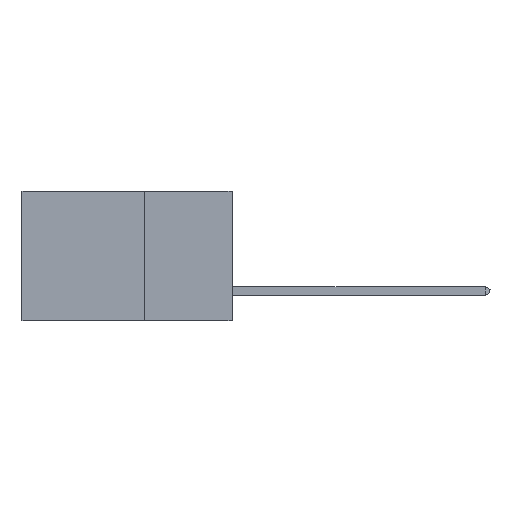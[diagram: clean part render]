
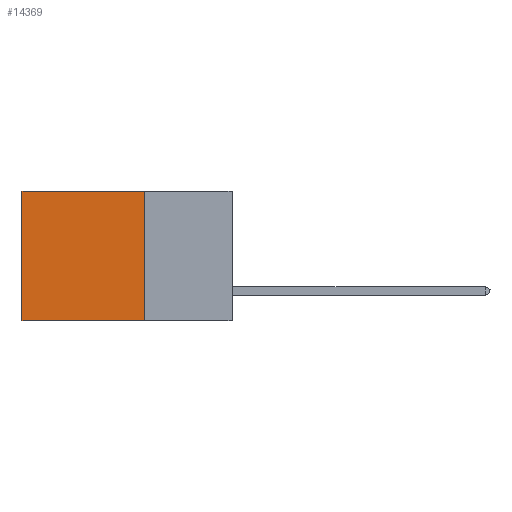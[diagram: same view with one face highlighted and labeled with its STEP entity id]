
A CAD part, left-side view. The second image highlights one B-rep face of the part: STEP entity #14369.
In plain terms, the highlighted planar face has unit normal (-1, 0, 0).
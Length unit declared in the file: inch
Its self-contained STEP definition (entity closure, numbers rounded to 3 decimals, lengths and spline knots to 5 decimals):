
#57 = CARTESIAN_POINT ( 'NONE',  ( 0.2875, 0.6, 0. ) ) ;
#259 = LINE ( 'NONE', #6716, #27695 ) ;
#378 = VERTEX_POINT ( 'NONE', #25871 ) ;
#605 = ORIENTED_EDGE ( 'NONE', *, *, #3742, .T. ) ;
#848 = LINE ( 'NONE', #57, #15889 ) ;
#2392 = EDGE_CURVE ( 'NONE', #14755, #378, #259, .T. ) ;
#3742 = EDGE_CURVE ( 'NONE', #21293, #25082, #848, .T. ) ;
#3989 = EDGE_LOOP ( 'NONE', ( #605, #13541, #4069, #24376 ) ) ;
#4069 = ORIENTED_EDGE ( 'NONE', *, *, #2392, .F. ) ;
#5235 = DIRECTION ( 'NONE',  ( 0., 1., 0. ) ) ;
#6046 = EDGE_CURVE ( 'NONE', #14755, #21293, #24447, .T. ) ;
#6399 = VECTOR ( 'NONE', #5235, 39.37008 ) ;
#6716 = CARTESIAN_POINT ( 'NONE',  ( 0.2875, 0.25, 0. ) ) ;
#7683 = DIRECTION ( 'NONE',  ( 0., 0., -1. ) ) ;
#9267 = DIRECTION ( 'NONE',  ( 0., 1., 0. ) ) ;
#9993 = VECTOR ( 'NONE', #9267, 39.37008 ) ;
#11596 = CARTESIAN_POINT ( 'NONE',  ( 0.2875, 0.25, 0. ) ) ;
#13541 = ORIENTED_EDGE ( 'NONE', *, *, #14747, .F. ) ;
#14369 = ADVANCED_FACE ( 'NONE', ( #18297 ), #20375, .F. ) ;
#14708 = CARTESIAN_POINT ( 'NONE',  ( 0.2875, 0.6, 0. ) ) ;
#14747 = EDGE_CURVE ( 'NONE', #378, #25082, #24338, .T. ) ;
#14755 = VERTEX_POINT ( 'NONE', #25963 ) ;
#15025 = DIRECTION ( 'NONE',  ( 0., 0., -1. ) ) ;
#15350 = CARTESIAN_POINT ( 'NONE',  ( 0.2875, 0.6, -0.37 ) ) ;
#15889 = VECTOR ( 'NONE', #15025, 39.37008 ) ;
#17629 = DIRECTION ( 'NONE',  ( 0., 0., -1. ) ) ;
#18297 = FACE_OUTER_BOUND ( 'NONE', #3989, .T. ) ;
#19886 = AXIS2_PLACEMENT_3D ( 'NONE', #22415, #20457, #7683 ) ;
#20375 = PLANE ( 'NONE',  #19886 ) ;
#20457 = DIRECTION ( 'NONE',  ( 1., 0., 0. ) ) ;
#21293 = VERTEX_POINT ( 'NONE', #14708 ) ;
#21661 = CARTESIAN_POINT ( 'NONE',  ( 0.2875, 0.25, -0.37 ) ) ;
#22415 = CARTESIAN_POINT ( 'NONE',  ( 0.2875, 0.25, 0. ) ) ;
#24338 = LINE ( 'NONE', #21661, #9993 ) ;
#24376 = ORIENTED_EDGE ( 'NONE', *, *, #6046, .T. ) ;
#24447 = LINE ( 'NONE', #11596, #6399 ) ;
#25082 = VERTEX_POINT ( 'NONE', #15350 ) ;
#25871 = CARTESIAN_POINT ( 'NONE',  ( 0.2875, 0.25, -0.37 ) ) ;
#25963 = CARTESIAN_POINT ( 'NONE',  ( 0.2875, 0.25, 0. ) ) ;
#27695 = VECTOR ( 'NONE', #17629, 39.37008 ) ;
